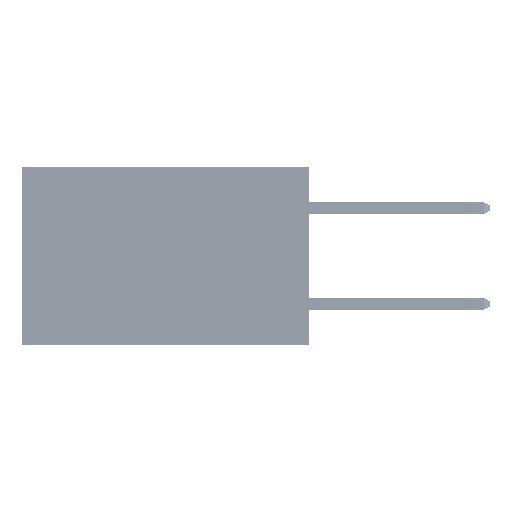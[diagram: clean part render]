
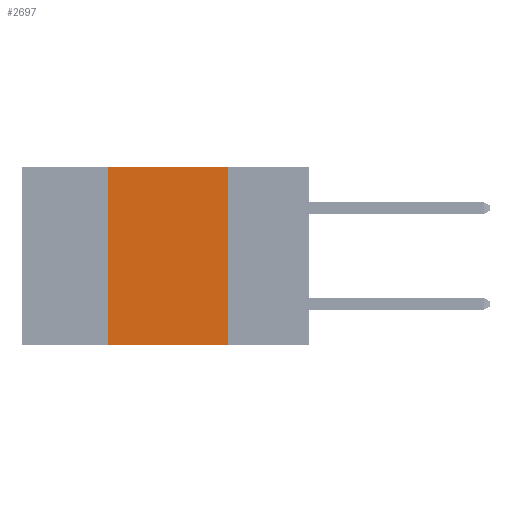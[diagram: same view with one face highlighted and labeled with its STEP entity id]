
A CAD part, left-side view. The second image highlights one B-rep face of the part: STEP entity #2697.
In plain terms, the highlighted planar face has unit normal (-1, 0, 0).
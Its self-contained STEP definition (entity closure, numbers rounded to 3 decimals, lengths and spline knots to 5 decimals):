
#2697 = ADVANCED_FACE ( 'NONE', ( #8900 ), #39552, .F. ) ;
#4428 = EDGE_CURVE ( 'NONE', #4866, #49389, #43358, .T. ) ;
#4866 = VERTEX_POINT ( 'NONE', #8282 ) ;
#5029 = DIRECTION ( 'NONE',  ( 0., -1., 0. ) ) ;
#6137 = EDGE_CURVE ( 'NONE', #23324, #6166, #46877, .T. ) ;
#6166 = VERTEX_POINT ( 'NONE', #38958 ) ;
#6230 = VECTOR ( 'NONE', #47887, 39.37008 ) ;
#6656 = VECTOR ( 'NONE', #8869, 39.37008 ) ;
#7358 = VECTOR ( 'NONE', #5029, 39.37008 ) ;
#8282 = CARTESIAN_POINT ( 'NONE',  ( 0., 0.42, -0.37 ) ) ;
#8507 = ORIENTED_EDGE ( 'NONE', *, *, #10933, .F. ) ;
#8869 = DIRECTION ( 'NONE',  ( 0., 0., -1. ) ) ;
#8900 = FACE_OUTER_BOUND ( 'NONE', #11451, .T. ) ;
#10933 = EDGE_CURVE ( 'NONE', #4866, #23324, #45916, .T. ) ;
#11451 = EDGE_LOOP ( 'NONE', ( #47456, #29763, #8507, #17747 ) ) ;
#16759 = CARTESIAN_POINT ( 'NONE',  ( 0., 0.6, -0.37 ) ) ;
#17747 = ORIENTED_EDGE ( 'NONE', *, *, #4428, .T. ) ;
#20141 = DIRECTION ( 'NONE',  ( 1., 0., 0. ) ) ;
#20636 = CARTESIAN_POINT ( 'NONE',  ( 0., 0.6, 0. ) ) ;
#21918 = CARTESIAN_POINT ( 'NONE',  ( 0., 0.42, 0. ) ) ;
#23324 = VERTEX_POINT ( 'NONE', #33031 ) ;
#29763 = ORIENTED_EDGE ( 'NONE', *, *, #6137, .F. ) ;
#31600 = AXIS2_PLACEMENT_3D ( 'NONE', #20636, #20141, #35236 ) ;
#32303 = CARTESIAN_POINT ( 'NONE',  ( 0., 0.6, 0. ) ) ;
#33031 = CARTESIAN_POINT ( 'NONE',  ( 0., 0.42, 0. ) ) ;
#35236 = DIRECTION ( 'NONE',  ( 0., 0., -1. ) ) ;
#37256 = DIRECTION ( 'NONE',  ( 0., 0., 1. ) ) ;
#38958 = CARTESIAN_POINT ( 'NONE',  ( 0., 0.17, 0. ) ) ;
#39552 = PLANE ( 'NONE',  #31600 ) ;
#40281 = LINE ( 'NONE', #47211, #6656 ) ;
#42645 = CARTESIAN_POINT ( 'NONE',  ( 0., 0.17, -0.37 ) ) ;
#42836 = EDGE_CURVE ( 'NONE', #6166, #49389, #40281, .T. ) ;
#43358 = LINE ( 'NONE', #16759, #7358 ) ;
#45916 = LINE ( 'NONE', #21918, #48714 ) ;
#46877 = LINE ( 'NONE', #32303, #6230 ) ;
#47211 = CARTESIAN_POINT ( 'NONE',  ( 0., 0.17, 0. ) ) ;
#47456 = ORIENTED_EDGE ( 'NONE', *, *, #42836, .F. ) ;
#47887 = DIRECTION ( 'NONE',  ( 0., -1., 0. ) ) ;
#48714 = VECTOR ( 'NONE', #37256, 39.37008 ) ;
#49389 = VERTEX_POINT ( 'NONE', #42645 ) ;
